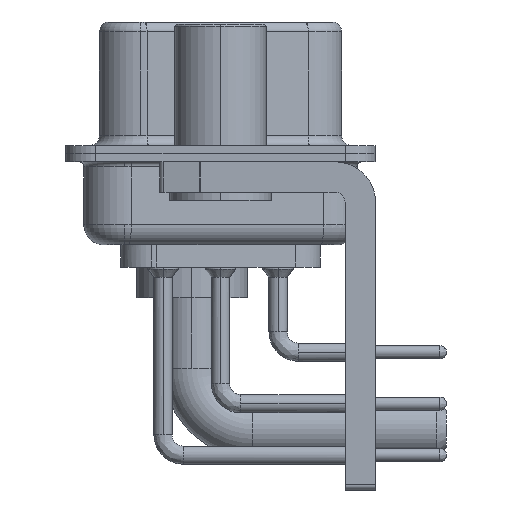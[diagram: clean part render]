
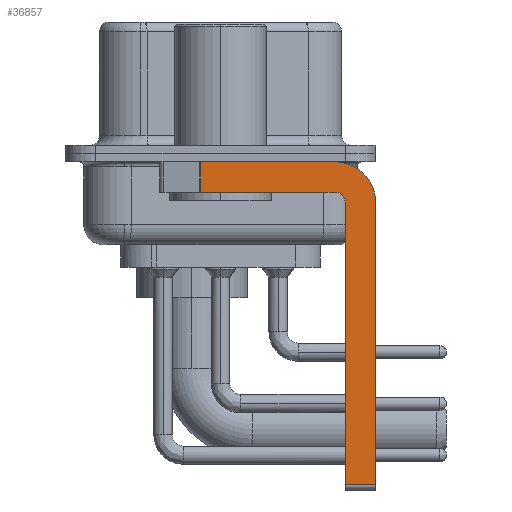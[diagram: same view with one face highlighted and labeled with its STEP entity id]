
A CAD part, left-side view. The second image highlights one B-rep face of the part: STEP entity #36857.
In plain terms, the highlighted planar face has unit normal (-1, 0, 0).
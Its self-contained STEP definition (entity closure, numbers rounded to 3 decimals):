
#2427 = FACE_OUTER_BOUND ( 'NONE', #3798, .T. ) ;
#3107 = DIRECTION ( 'NONE',  ( 0., 0., -1. ) ) ;
#3683 = VERTEX_POINT ( 'NONE', #27733 ) ;
#3798 = EDGE_LOOP ( 'NONE', ( #32472, #33328, #21347, #20665, #35836, #12304, #22813, #27026 ) ) ;
#4540 = VERTEX_POINT ( 'NONE', #33710 ) ;
#4863 = EDGE_CURVE ( 'NONE', #4540, #21021, #17023, .T. ) ;
#5743 = CIRCLE ( 'NONE', #18280, 2. ) ;
#6000 = DIRECTION ( 'NONE',  ( 0., 0., 1. ) ) ;
#6278 = CARTESIAN_POINT ( 'NONE',  ( -2.9, 3., -0.4 ) ) ;
#6459 = DIRECTION ( 'NONE',  ( 1., 0., 0. ) ) ;
#7413 = VECTOR ( 'NONE', #29527, 1000. ) ;
#7680 = VECTOR ( 'NONE', #7682, 1000. ) ;
#7682 = DIRECTION ( 'NONE',  ( 0., 0., -1. ) ) ;
#8555 = DIRECTION ( 'NONE',  ( -1., 0., 0. ) ) ;
#8733 = LINE ( 'NONE', #15228, #29227 ) ;
#9117 = CARTESIAN_POINT ( 'NONE',  ( -2.9, -7.65, -16.35 ) ) ;
#9275 = LINE ( 'NONE', #15375, #30619 ) ;
#9295 = CARTESIAN_POINT ( 'NONE',  ( -2.9, -5.65, -1.9 ) ) ;
#9943 = AXIS2_PLACEMENT_3D ( 'NONE', #27142, #21064, #17529 ) ;
#12098 = LINE ( 'NONE', #26599, #7413 ) ;
#12118 = VERTEX_POINT ( 'NONE', #38125 ) ;
#12184 = VERTEX_POINT ( 'NONE', #15756 ) ;
#12274 = EDGE_CURVE ( 'NONE', #3683, #22496, #9275, .T. ) ;
#12304 = ORIENTED_EDGE ( 'NONE', *, *, #12274, .T. ) ;
#13419 = VERTEX_POINT ( 'NONE', #35163 ) ;
#14961 = CARTESIAN_POINT ( 'NONE',  ( -2.9, 0.978, -0.4 ) ) ;
#15023 = CIRCLE ( 'NONE', #30670, 0.5 ) ;
#15228 = CARTESIAN_POINT ( 'NONE',  ( -2.9, -6.15, -16.6 ) ) ;
#15375 = CARTESIAN_POINT ( 'NONE',  ( -2.9, -5.65, -16.35 ) ) ;
#15756 = CARTESIAN_POINT ( 'NONE',  ( -2.9, -7.65, -2.4 ) ) ;
#16714 = CARTESIAN_POINT ( 'NONE',  ( -2.9, -7.65, -2.4 ) ) ;
#17023 = LINE ( 'NONE', #9295, #26320 ) ;
#17529 = DIRECTION ( 'NONE',  ( 0., 0., -1. ) ) ;
#17807 = VERTEX_POINT ( 'NONE', #14961 ) ;
#18052 = EDGE_CURVE ( 'NONE', #12184, #22496, #19101, .T. ) ;
#18280 = AXIS2_PLACEMENT_3D ( 'NONE', #24297, #6459, #3107 ) ;
#19101 = LINE ( 'NONE', #16714, #7680 ) ;
#20438 = CARTESIAN_POINT ( 'NONE',  ( -2.9, 0.978, -1.9 ) ) ;
#20533 = VECTOR ( 'NONE', #32547, 1000. ) ;
#20665 = ORIENTED_EDGE ( 'NONE', *, *, #25525, .F. ) ;
#20719 = DIRECTION ( 'NONE',  ( 0., 0., 1. ) ) ;
#21021 = VERTEX_POINT ( 'NONE', #20438 ) ;
#21064 = DIRECTION ( 'NONE',  ( 1., 0., 0. ) ) ;
#21347 = ORIENTED_EDGE ( 'NONE', *, *, #4863, .F. ) ;
#22496 = VERTEX_POINT ( 'NONE', #9117 ) ;
#22813 = ORIENTED_EDGE ( 'NONE', *, *, #18052, .F. ) ;
#23416 = EDGE_CURVE ( 'NONE', #17807, #13419, #23722, .T. ) ;
#23722 = LINE ( 'NONE', #6278, #20533 ) ;
#23841 = CARTESIAN_POINT ( 'NONE',  ( -2.9, -5.65, -2.4 ) ) ;
#24297 = CARTESIAN_POINT ( 'NONE',  ( -2.9, -5.65, -2.4 ) ) ;
#24585 = DIRECTION ( 'NONE',  ( 0., -1., 0. ) ) ;
#25525 = EDGE_CURVE ( 'NONE', #12118, #4540, #15023, .T. ) ;
#26320 = VECTOR ( 'NONE', #35763, 1000. ) ;
#26356 = PLANE ( 'NONE',  #9943 ) ;
#26599 = CARTESIAN_POINT ( 'NONE',  ( -2.9, 0.978, -1.9 ) ) ;
#27026 = ORIENTED_EDGE ( 'NONE', *, *, #28928, .F. ) ;
#27142 = CARTESIAN_POINT ( 'NONE',  ( -2.9, -5.65, -2.4 ) ) ;
#27733 = CARTESIAN_POINT ( 'NONE',  ( -2.9, -6.15, -16.35 ) ) ;
#28928 = EDGE_CURVE ( 'NONE', #13419, #12184, #5743, .T. ) ;
#29227 = VECTOR ( 'NONE', #6000, 1000. ) ;
#29527 = DIRECTION ( 'NONE',  ( 0., 0., -1. ) ) ;
#30619 = VECTOR ( 'NONE', #24585, 1000. ) ;
#30670 = AXIS2_PLACEMENT_3D ( 'NONE', #23841, #8555, #20719 ) ;
#32472 = ORIENTED_EDGE ( 'NONE', *, *, #23416, .F. ) ;
#32547 = DIRECTION ( 'NONE',  ( 0., -1., 0. ) ) ;
#33328 = ORIENTED_EDGE ( 'NONE', *, *, #36540, .T. ) ;
#33710 = CARTESIAN_POINT ( 'NONE',  ( -2.9, -5.65, -1.9 ) ) ;
#35124 = EDGE_CURVE ( 'NONE', #3683, #12118, #8733, .T. ) ;
#35163 = CARTESIAN_POINT ( 'NONE',  ( -2.9, -5.65, -0.4 ) ) ;
#35763 = DIRECTION ( 'NONE',  ( 0., 1., 0. ) ) ;
#35836 = ORIENTED_EDGE ( 'NONE', *, *, #35124, .F. ) ;
#36540 = EDGE_CURVE ( 'NONE', #17807, #21021, #12098, .T. ) ;
#36857 = ADVANCED_FACE ( 'NONE', ( #2427 ), #26356, .F. ) ;
#38125 = CARTESIAN_POINT ( 'NONE',  ( -2.9, -6.15, -2.4 ) ) ;
